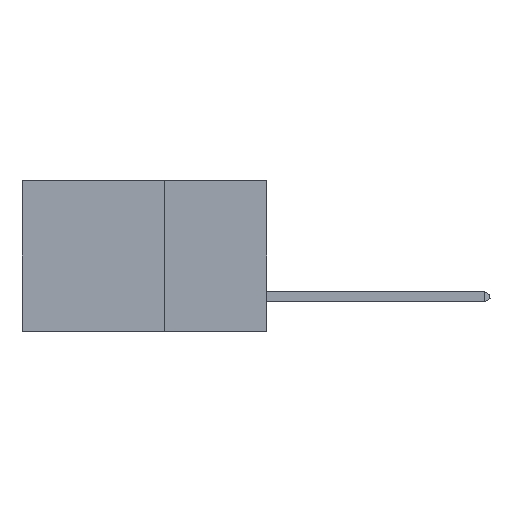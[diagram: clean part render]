
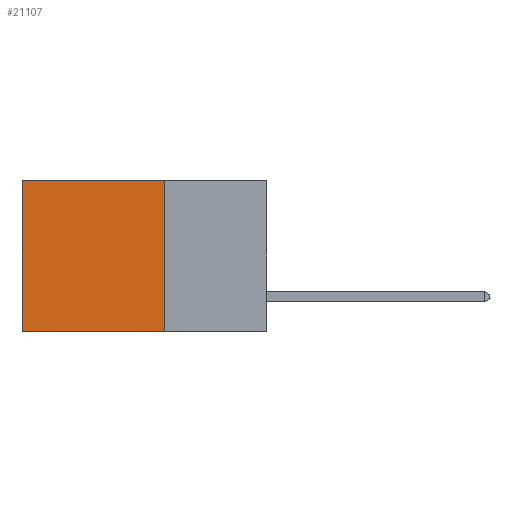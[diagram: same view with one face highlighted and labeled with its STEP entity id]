
A CAD part, left-side view. The second image highlights one B-rep face of the part: STEP entity #21107.
In plain terms, the highlighted planar face has unit normal (-1, 0, 0).
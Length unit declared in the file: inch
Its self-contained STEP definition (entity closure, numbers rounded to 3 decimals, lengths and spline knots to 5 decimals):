
#1699 = ORIENTED_EDGE ( 'NONE', *, *, #26259, .F. ) ;
#1866 = VECTOR ( 'NONE', #27595, 39.37008 ) ;
#2335 = DIRECTION ( 'NONE',  ( 1., 0., 0. ) ) ;
#2740 = CARTESIAN_POINT ( 'NONE',  ( 0.2875, 0.25, 0. ) ) ;
#2851 = VERTEX_POINT ( 'NONE', #18879 ) ;
#3399 = DIRECTION ( 'NONE',  ( 0., 0., -1. ) ) ;
#4326 = CARTESIAN_POINT ( 'NONE',  ( 0.2875, 0.6, -0.37 ) ) ;
#4880 = DIRECTION ( 'NONE',  ( 0., 1., 0. ) ) ;
#5102 = CARTESIAN_POINT ( 'NONE',  ( 0.2875, 0.6, 0. ) ) ;
#7495 = FACE_OUTER_BOUND ( 'NONE', #17983, .T. ) ;
#8394 = DIRECTION ( 'NONE',  ( 0., 0., -1. ) ) ;
#8600 = LINE ( 'NONE', #40890, #35590 ) ;
#11195 = EDGE_CURVE ( 'NONE', #25331, #28032, #20357, .T. ) ;
#11905 = CARTESIAN_POINT ( 'NONE',  ( 0.2875, 0.25, 0. ) ) ;
#12891 = VERTEX_POINT ( 'NONE', #11905 ) ;
#17197 = VECTOR ( 'NONE', #40084, 39.37008 ) ;
#17983 = EDGE_LOOP ( 'NONE', ( #34127, #31165, #1699, #23933 ) ) ;
#18879 = CARTESIAN_POINT ( 'NONE',  ( 0.2875, 0.25, -0.37 ) ) ;
#19679 = LINE ( 'NONE', #40222, #17197 ) ;
#20357 = LINE ( 'NONE', #5102, #1866 ) ;
#20723 = VECTOR ( 'NONE', #4880, 39.37008 ) ;
#21107 = ADVANCED_FACE ( 'NONE', ( #7495 ), #28059, .F. ) ;
#21228 = LINE ( 'NONE', #37215, #20723 ) ;
#23933 = ORIENTED_EDGE ( 'NONE', *, *, #30245, .T. ) ;
#25228 = EDGE_CURVE ( 'NONE', #2851, #28032, #21228, .T. ) ;
#25331 = VERTEX_POINT ( 'NONE', #26269 ) ;
#26259 = EDGE_CURVE ( 'NONE', #12891, #2851, #8600, .T. ) ;
#26269 = CARTESIAN_POINT ( 'NONE',  ( 0.2875, 0.6, 0. ) ) ;
#27595 = DIRECTION ( 'NONE',  ( 0., 0., -1. ) ) ;
#28032 = VERTEX_POINT ( 'NONE', #4326 ) ;
#28059 = PLANE ( 'NONE',  #29874 ) ;
#29874 = AXIS2_PLACEMENT_3D ( 'NONE', #2740, #2335, #3399 ) ;
#30245 = EDGE_CURVE ( 'NONE', #12891, #25331, #19679, .T. ) ;
#31165 = ORIENTED_EDGE ( 'NONE', *, *, #25228, .F. ) ;
#34127 = ORIENTED_EDGE ( 'NONE', *, *, #11195, .T. ) ;
#35590 = VECTOR ( 'NONE', #8394, 39.37008 ) ;
#37215 = CARTESIAN_POINT ( 'NONE',  ( 0.2875, 0.25, -0.37 ) ) ;
#40084 = DIRECTION ( 'NONE',  ( 0., 1., 0. ) ) ;
#40222 = CARTESIAN_POINT ( 'NONE',  ( 0.2875, 0.25, 0. ) ) ;
#40890 = CARTESIAN_POINT ( 'NONE',  ( 0.2875, 0.25, 0. ) ) ;
